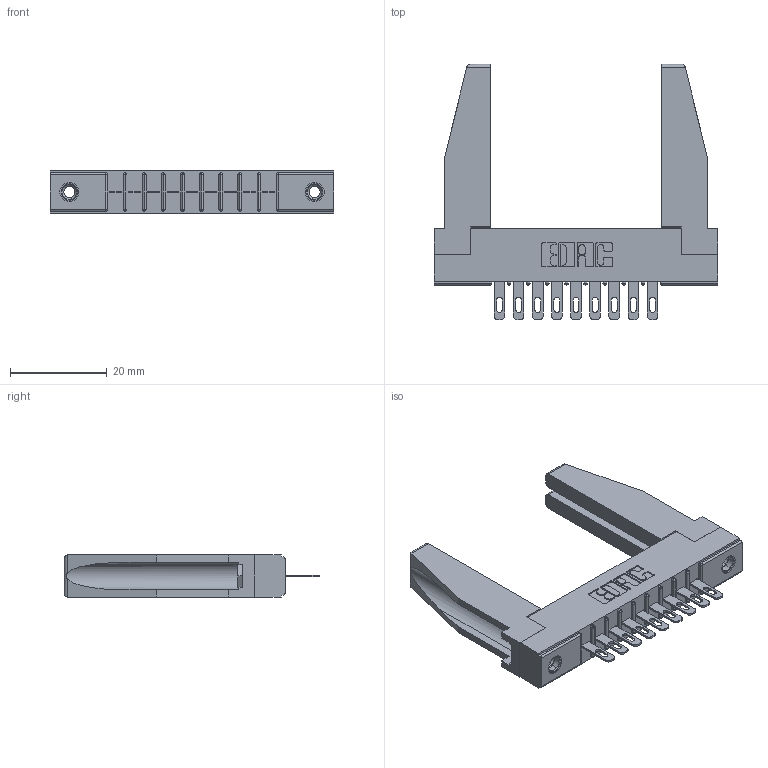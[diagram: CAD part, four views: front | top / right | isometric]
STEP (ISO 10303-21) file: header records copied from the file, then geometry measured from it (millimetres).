
FILE_DESCRIPTION (( 'STEP AP203' ), '1' );
FILE_NAME ('356-009-400-178.STEP', '2020-09-23T09:31:07', ( '' ), ( '' ), 'SwSTEP 2.0', 'SolidWorks 2020', '' );
FILE_SCHEMA (( 'CONFIG_CONTROL_DESIGN' ));
Length unit declared in the file: inch
Products named in the file (5): 356-009-400-178; 345-250-001_345-250-001-102; 307-220-078; 306-290-001_100; 306 Part_.156 Dia
Assembly tree (14 placements, depth 2):
  356-009-400-178
    306 Part_.156 Dia
    306-290-001_100  x9
    345-250-001_345-250-001-102  x2
    307-220-078  x2
Bounding box: 58.67 x 52.91 x 8.71 mm (x, y, z)
Volume: 7973.8 mm3; surface area: 9457.1 mm2
Topology: 14 solids, 14 shells, 930 faces, 2581 edges, 1662 vertices
Faces by surface type: plane 602, cylinder 276, sphere 36, cone 12, torus 4
Entity records: 15271 total; most frequent: CARTESIAN_POINT 2560, ORIENTED_EDGE 2492, DIRECTION 2480, EDGE_CURVE 1246, LINE 956, VECTOR 956, VERTEX_POINT 800, AXIS2_PLACEMENT_3D 762
